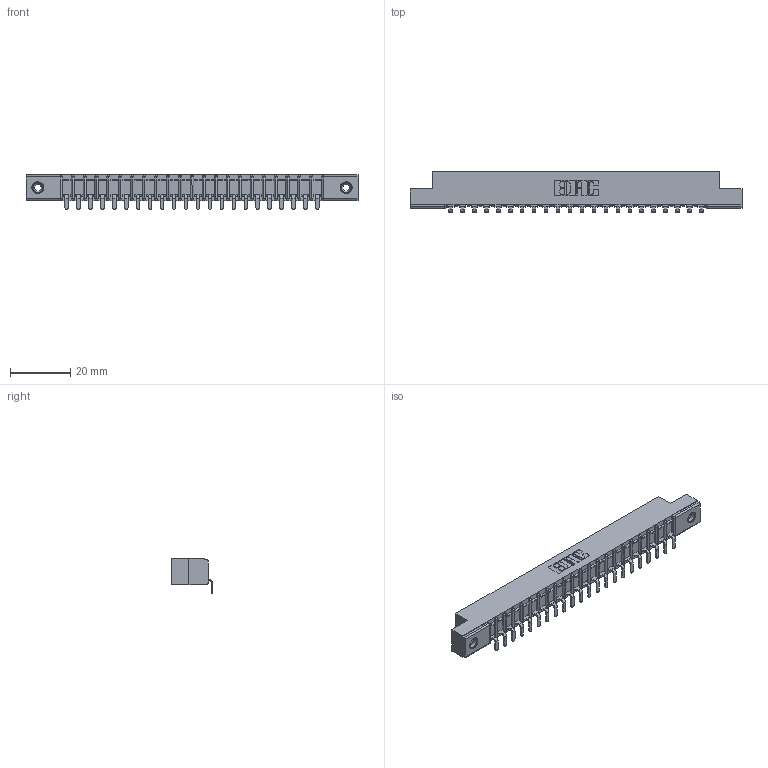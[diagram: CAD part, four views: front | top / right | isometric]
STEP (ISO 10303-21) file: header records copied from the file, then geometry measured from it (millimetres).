
FILE_DESCRIPTION (( 'STEP AP203' ), '1' );
FILE_NAME ('357-022-553-108.STEP', '2019-09-16T23:18:16', ( '' ), ( '' ), 'SwSTEP 2.0', 'SolidWorks 2016', '' );
FILE_SCHEMA (( 'CONFIG_CONTROL_DESIGN' ));
Length unit declared in the file: inch
Products named in the file (4): 345-250-001_345-250-003-102; 307-290-002_553; 307 Part_.156 Dia Mounting Holes; 357-022-553-108
Assembly tree (25 placements, depth 2):
  357-022-553-108
    307 Part_.156 Dia Mounting Holes
    307-290-002_553  x22
    345-250-001_345-250-003-102  x2
Bounding box: 110.19 x 13.32 x 11.51 mm (x, y, z)
Volume: 7267.6 mm3; surface area: 13243.9 mm2
Topology: 25 solids, 25 shells, 1917 faces, 5827 edges, 3814 vertices
Faces by surface type: plane 1136, cylinder 719, sphere 46, cone 12, torus 4
Entity records: 23365 total; most frequent: CARTESIAN_POINT 3919, ORIENTED_EDGE 3902, DIRECTION 3827, EDGE_CURVE 1951, VECTOR 1483, LINE 1483, VERTEX_POINT 1264, AXIS2_PLACEMENT_3D 1172
